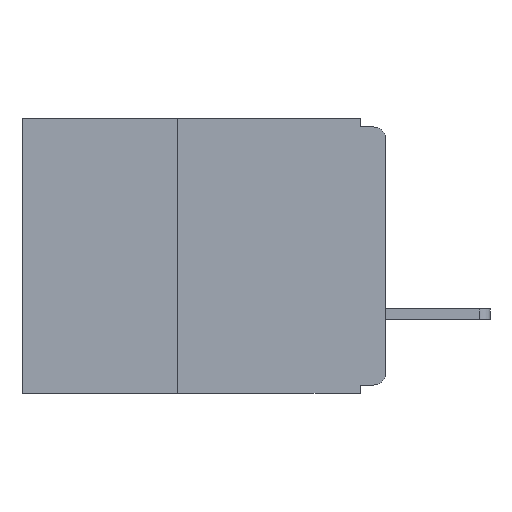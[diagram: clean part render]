
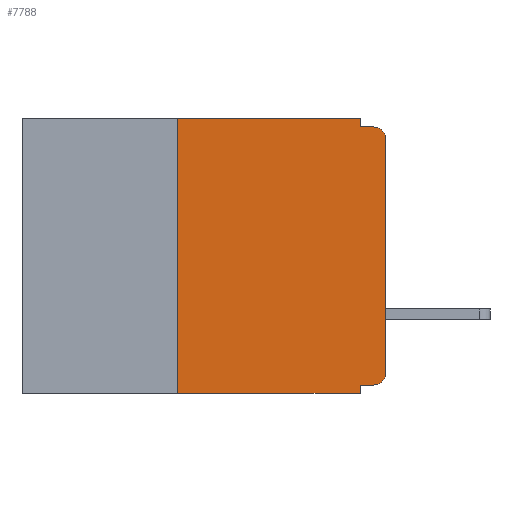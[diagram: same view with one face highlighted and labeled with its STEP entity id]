
A CAD part, left-side view. The second image highlights one B-rep face of the part: STEP entity #7788.
In plain terms, the highlighted planar face has unit normal (-1, 0, 0).
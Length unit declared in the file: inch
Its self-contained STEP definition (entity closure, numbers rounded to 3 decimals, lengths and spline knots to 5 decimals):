
#52 = CARTESIAN_POINT ( 'NONE',  ( 0., 0.25, -0.33 ) ) ;
#190 = DIRECTION ( 'NONE',  ( 0., 0., 1. ) ) ;
#252 = EDGE_LOOP ( 'NONE', ( #2866, #5372, #17586, #2650, #18180, #19977, #11457, #27971, #7581, #6664 ) ) ;
#341 = VECTOR ( 'NONE', #25610, 39.37008 ) ;
#867 = CARTESIAN_POINT ( 'NONE',  ( 0., 0., -0.32 ) ) ;
#2650 = ORIENTED_EDGE ( 'NONE', *, *, #13528, .F. ) ;
#2866 = ORIENTED_EDGE ( 'NONE', *, *, #4740, .T. ) ;
#3249 = VERTEX_POINT ( 'NONE', #29044 ) ;
#3400 = CARTESIAN_POINT ( 'NONE',  ( 0., 0.031, -0.32 ) ) ;
#4209 = DIRECTION ( 'NONE',  ( 0., -1., 0. ) ) ;
#4740 = EDGE_CURVE ( 'NONE', #27307, #6080, #22027, .T. ) ;
#5039 = EDGE_CURVE ( 'NONE', #6847, #5342, #7259, .T. ) ;
#5222 = DIRECTION ( 'NONE',  ( 0., 0., 1. ) ) ;
#5342 = VERTEX_POINT ( 'NONE', #13469 ) ;
#5372 = ORIENTED_EDGE ( 'NONE', *, *, #26593, .T. ) ;
#5673 = EDGE_CURVE ( 'NONE', #3249, #23711, #33604, .T. ) ;
#6080 = VERTEX_POINT ( 'NONE', #16333 ) ;
#6274 = CARTESIAN_POINT ( 'NONE',  ( 0., 0.031, -0.01 ) ) ;
#6301 = EDGE_CURVE ( 'NONE', #8553, #29198, #27756, .T. ) ;
#6664 = ORIENTED_EDGE ( 'NONE', *, *, #15167, .T. ) ;
#6756 = CARTESIAN_POINT ( 'NONE',  ( 0., 0.031, 0. ) ) ;
#6847 = VERTEX_POINT ( 'NONE', #17074 ) ;
#7148 = LINE ( 'NONE', #27104, #8003 ) ;
#7259 = LINE ( 'NONE', #12194, #19847 ) ;
#7581 = ORIENTED_EDGE ( 'NONE', *, *, #5673, .F. ) ;
#7689 = VECTOR ( 'NONE', #5222, 39.37008 ) ;
#7788 = ADVANCED_FACE ( 'NONE', ( #28074 ), #21660, .F. ) ;
#7862 = CARTESIAN_POINT ( 'NONE',  ( 0., 0.015, -0.01 ) ) ;
#8003 = VECTOR ( 'NONE', #29749, 39.37008 ) ;
#8553 = VERTEX_POINT ( 'NONE', #6274 ) ;
#8593 = EDGE_CURVE ( 'NONE', #23711, #22132, #30492, .T. ) ;
#9244 = CARTESIAN_POINT ( 'NONE',  ( 0., 0., -0.01 ) ) ;
#9344 = LINE ( 'NONE', #52, #7689 ) ;
#10490 = AXIS2_PLACEMENT_3D ( 'NONE', #31220, #15141, #33877 ) ;
#10555 = CARTESIAN_POINT ( 'NONE',  ( 0., 0.015, -0.305 ) ) ;
#10887 = DIRECTION ( 'NONE',  ( 0., 0., -1. ) ) ;
#11457 = ORIENTED_EDGE ( 'NONE', *, *, #33161, .T. ) ;
#12177 = VECTOR ( 'NONE', #17156, 39.37008 ) ;
#12194 = CARTESIAN_POINT ( 'NONE',  ( 0., 0.437, 0. ) ) ;
#13224 = DIRECTION ( 'NONE',  ( 0., 0., -1. ) ) ;
#13469 = CARTESIAN_POINT ( 'NONE',  ( 0., 0.031, 0. ) ) ;
#13528 = EDGE_CURVE ( 'NONE', #5342, #8553, #34550, .T. ) ;
#13915 = EDGE_CURVE ( 'NONE', #32202, #6847, #9344, .T. ) ;
#14472 = CARTESIAN_POINT ( 'NONE',  ( 0., 0.031, -0.33 ) ) ;
#15141 = DIRECTION ( 'NONE',  ( -1., 0., 0. ) ) ;
#15167 = EDGE_CURVE ( 'NONE', #3249, #27307, #30655, .T. ) ;
#16333 = CARTESIAN_POINT ( 'NONE',  ( 0., 0., -0.025 ) ) ;
#17062 = VECTOR ( 'NONE', #30460, 39.37008 ) ;
#17074 = CARTESIAN_POINT ( 'NONE',  ( 0., 0.25, 0. ) ) ;
#17156 = DIRECTION ( 'NONE',  ( 0., 1., 0. ) ) ;
#17586 = ORIENTED_EDGE ( 'NONE', *, *, #6301, .F. ) ;
#18180 = ORIENTED_EDGE ( 'NONE', *, *, #5039, .F. ) ;
#19847 = VECTOR ( 'NONE', #4209, 39.37008 ) ;
#19977 = ORIENTED_EDGE ( 'NONE', *, *, #13915, .F. ) ;
#19985 = CARTESIAN_POINT ( 'NONE',  ( 0., 0.25, -0.33 ) ) ;
#20067 = DIRECTION ( 'NONE',  ( 0., -1., 0. ) ) ;
#20628 = VECTOR ( 'NONE', #20067, 39.37008 ) ;
#21660 = PLANE ( 'NONE',  #24647 ) ;
#21956 = CARTESIAN_POINT ( 'NONE',  ( 0., 0., 0. ) ) ;
#22027 = LINE ( 'NONE', #21956, #29115 ) ;
#22132 = VERTEX_POINT ( 'NONE', #25228 ) ;
#23579 = CIRCLE ( 'NONE', #10490, 0.015 ) ;
#23711 = VERTEX_POINT ( 'NONE', #3400 ) ;
#24647 = AXIS2_PLACEMENT_3D ( 'NONE', #34940, #27038, #10887 ) ;
#25228 = CARTESIAN_POINT ( 'NONE',  ( 0., 0.031, -0.33 ) ) ;
#25610 = DIRECTION ( 'NONE',  ( 0., 0., -1. ) ) ;
#26311 = CARTESIAN_POINT ( 'NONE',  ( 0., 0., -0.305 ) ) ;
#26593 = EDGE_CURVE ( 'NONE', #6080, #29198, #23579, .T. ) ;
#27038 = DIRECTION ( 'NONE',  ( 1., 0., 0. ) ) ;
#27104 = CARTESIAN_POINT ( 'NONE',  ( 0., 0.437, -0.33 ) ) ;
#27307 = VERTEX_POINT ( 'NONE', #26311 ) ;
#27756 = LINE ( 'NONE', #9244, #20628 ) ;
#27971 = ORIENTED_EDGE ( 'NONE', *, *, #8593, .F. ) ;
#28074 = FACE_OUTER_BOUND ( 'NONE', #252, .T. ) ;
#29044 = CARTESIAN_POINT ( 'NONE',  ( 0., 0.015, -0.32 ) ) ;
#29115 = VECTOR ( 'NONE', #190, 39.37008 ) ;
#29198 = VERTEX_POINT ( 'NONE', #7862 ) ;
#29268 = AXIS2_PLACEMENT_3D ( 'NONE', #10555, #29349, #13224 ) ;
#29349 = DIRECTION ( 'NONE',  ( -1., 0., 0. ) ) ;
#29749 = DIRECTION ( 'NONE',  ( 0., -1., 0. ) ) ;
#30460 = DIRECTION ( 'NONE',  ( 0., 0., -1. ) ) ;
#30492 = LINE ( 'NONE', #14472, #17062 ) ;
#30655 = CIRCLE ( 'NONE', #29268, 0.015 ) ;
#31220 = CARTESIAN_POINT ( 'NONE',  ( 0., 0.015, -0.025 ) ) ;
#32202 = VERTEX_POINT ( 'NONE', #19985 ) ;
#33161 = EDGE_CURVE ( 'NONE', #32202, #22132, #7148, .T. ) ;
#33604 = LINE ( 'NONE', #867, #12177 ) ;
#33877 = DIRECTION ( 'NONE',  ( 0., 0., -1. ) ) ;
#34550 = LINE ( 'NONE', #6756, #341 ) ;
#34940 = CARTESIAN_POINT ( 'NONE',  ( 0., 0.437, 0. ) ) ;
